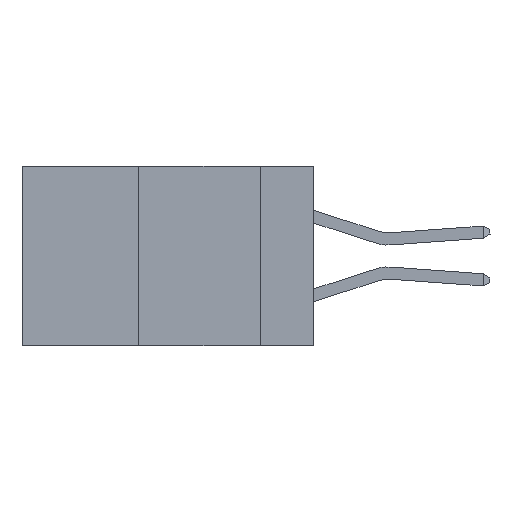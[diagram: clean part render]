
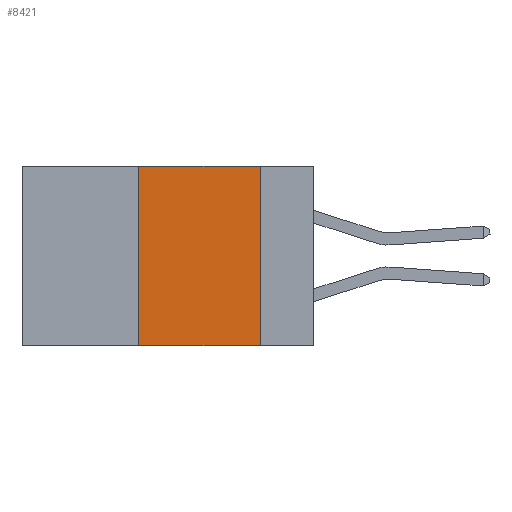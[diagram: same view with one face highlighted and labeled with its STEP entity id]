
A CAD part, left-side view. The second image highlights one B-rep face of the part: STEP entity #8421.
In plain terms, the highlighted planar face has unit normal (-1, 0, 0).
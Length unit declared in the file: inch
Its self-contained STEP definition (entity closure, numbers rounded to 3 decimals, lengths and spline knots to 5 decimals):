
#44 = LINE ( 'NONE', #4993, #5062 ) ;
#668 = DIRECTION ( 'NONE',  ( 0., -1., 0. ) ) ;
#809 = VERTEX_POINT ( 'NONE', #16001 ) ;
#1585 = AXIS2_PLACEMENT_3D ( 'NONE', #20145, #22291, #10042 ) ;
#3783 = PLANE ( 'NONE',  #1585 ) ;
#3923 = CARTESIAN_POINT ( 'NONE',  ( 0., 0.11, -0.37 ) ) ;
#4081 = EDGE_LOOP ( 'NONE', ( #24267, #14734, #6350, #6686 ) ) ;
#4539 = VECTOR ( 'NONE', #668, 39.37008 ) ;
#4725 = VECTOR ( 'NONE', #25851, 39.37008 ) ;
#4993 = CARTESIAN_POINT ( 'NONE',  ( 0., 0.11, 0. ) ) ;
#5062 = VECTOR ( 'NONE', #13191, 39.37008 ) ;
#5499 = CARTESIAN_POINT ( 'NONE',  ( 0., 0.36, 0. ) ) ;
#6350 = ORIENTED_EDGE ( 'NONE', *, *, #12859, .F. ) ;
#6444 = EDGE_CURVE ( 'NONE', #23095, #7423, #9811, .T. ) ;
#6686 = ORIENTED_EDGE ( 'NONE', *, *, #10429, .T. ) ;
#7423 = VERTEX_POINT ( 'NONE', #23396 ) ;
#8421 = ADVANCED_FACE ( 'NONE', ( #10634 ), #3783, .F. ) ;
#9174 = VECTOR ( 'NONE', #24495, 39.37008 ) ;
#9777 = EDGE_CURVE ( 'NONE', #7423, #25946, #44, .T. ) ;
#9811 = LINE ( 'NONE', #12284, #9174 ) ;
#10042 = DIRECTION ( 'NONE',  ( 0., 0., -1. ) ) ;
#10046 = LINE ( 'NONE', #23174, #4539 ) ;
#10429 = EDGE_CURVE ( 'NONE', #809, #25946, #10046, .T. ) ;
#10634 = FACE_OUTER_BOUND ( 'NONE', #4081, .T. ) ;
#12284 = CARTESIAN_POINT ( 'NONE',  ( 0., 0.6, 0. ) ) ;
#12859 = EDGE_CURVE ( 'NONE', #809, #23095, #15053, .T. ) ;
#13191 = DIRECTION ( 'NONE',  ( 0., 0., -1. ) ) ;
#14734 = ORIENTED_EDGE ( 'NONE', *, *, #6444, .F. ) ;
#15053 = LINE ( 'NONE', #19739, #4725 ) ;
#16001 = CARTESIAN_POINT ( 'NONE',  ( 0., 0.36, -0.37 ) ) ;
#19739 = CARTESIAN_POINT ( 'NONE',  ( 0., 0.36, 0. ) ) ;
#20145 = CARTESIAN_POINT ( 'NONE',  ( 0., 0.6, 0. ) ) ;
#22291 = DIRECTION ( 'NONE',  ( 1., 0., 0. ) ) ;
#23095 = VERTEX_POINT ( 'NONE', #5499 ) ;
#23174 = CARTESIAN_POINT ( 'NONE',  ( 0., 0.6, -0.37 ) ) ;
#23396 = CARTESIAN_POINT ( 'NONE',  ( 0., 0.11, 0. ) ) ;
#24267 = ORIENTED_EDGE ( 'NONE', *, *, #9777, .F. ) ;
#24495 = DIRECTION ( 'NONE',  ( 0., -1., 0. ) ) ;
#25851 = DIRECTION ( 'NONE',  ( 0., 0., 1. ) ) ;
#25946 = VERTEX_POINT ( 'NONE', #3923 ) ;
